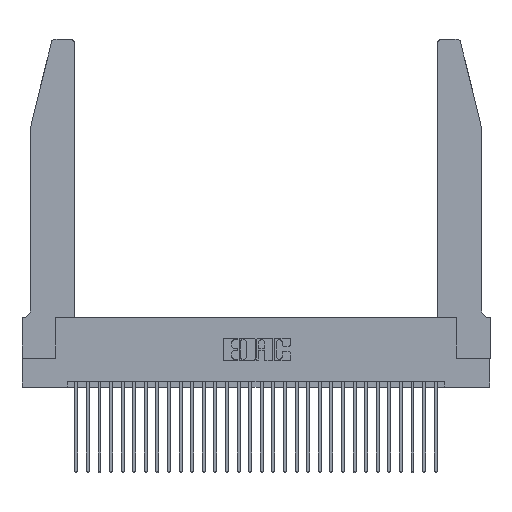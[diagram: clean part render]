
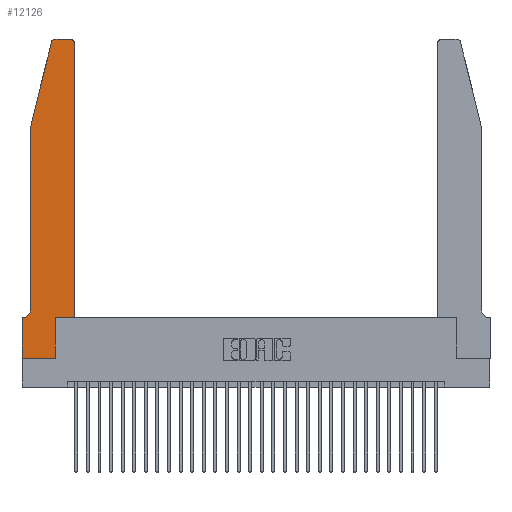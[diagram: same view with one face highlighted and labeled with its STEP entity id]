
A CAD part, top view. The second image highlights one B-rep face of the part: STEP entity #12126.
In plain terms, the highlighted planar face has unit normal (0, 0, 1).
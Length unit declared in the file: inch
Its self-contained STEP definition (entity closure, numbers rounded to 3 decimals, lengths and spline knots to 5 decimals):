
#45 = DIRECTION ( 'NONE',  ( 1., 0., 0. ) ) ;
#242 = DIRECTION ( 'NONE',  ( 1., 0., 0. ) ) ;
#439 = CARTESIAN_POINT ( 'NONE',  ( 0., 0., 0.37 ) ) ;
#577 = CARTESIAN_POINT ( 'NONE',  ( 0.0755, 0.35, 0.37 ) ) ;
#1180 = LINE ( 'NONE', #14344, #19770 ) ;
#1214 = EDGE_CURVE ( 'NONE', #13601, #24183, #5339, .T. ) ;
#1487 = CARTESIAN_POINT ( 'NONE',  ( 0.0755, 2., 0.37 ) ) ;
#1635 = CARTESIAN_POINT ( 'NONE',  ( 0.4205, 2.72, 0.37 ) ) ;
#1815 = EDGE_CURVE ( 'NONE', #28542, #14174, #22331, .T. ) ;
#2002 = EDGE_CURVE ( 'NONE', #27804, #28542, #4915, .T. ) ;
#2215 = CARTESIAN_POINT ( 'NONE',  ( 0.25487, 2.72718, 0.37 ) ) ;
#2487 = ORIENTED_EDGE ( 'NONE', *, *, #30683, .T. ) ;
#2909 = DIRECTION ( 'NONE',  ( 0., -1., 0. ) ) ;
#3044 = LINE ( 'NONE', #439, #27977 ) ;
#3140 = CARTESIAN_POINT ( 'NONE',  ( 0.2605, 2.75, 0.37 ) ) ;
#3738 = ORIENTED_EDGE ( 'NONE', *, *, #28276, .T. ) ;
#3820 = FACE_OUTER_BOUND ( 'NONE', #18249, .T. ) ;
#4070 = ORIENTED_EDGE ( 'NONE', *, *, #11507, .T. ) ;
#4106 = DIRECTION ( 'NONE',  ( 1., 0., 0. ) ) ;
#4196 = LINE ( 'NONE', #3140, #22747 ) ;
#4547 = CARTESIAN_POINT ( 'NONE',  ( 0.4505, 0.35, 0.37 ) ) ;
#4696 = VERTEX_POINT ( 'NONE', #9261 ) ;
#4725 = DIRECTION ( 'NONE',  ( 1., 0., 0. ) ) ;
#4732 = AXIS2_PLACEMENT_3D ( 'NONE', #1635, #18627, #4106 ) ;
#4915 = LINE ( 'NONE', #17251, #10599 ) ;
#5339 = LINE ( 'NONE', #577, #30224 ) ;
#5496 = CARTESIAN_POINT ( 'NONE',  ( 0.2865, 0.35, 0.37 ) ) ;
#5604 = DIRECTION ( 'NONE',  ( -1., 0., 0. ) ) ;
#5750 = CARTESIAN_POINT ( 'NONE',  ( 0.0055, 0.42, 0.37 ) ) ;
#5831 = EDGE_CURVE ( 'NONE', #15368, #27804, #14649, .T. ) ;
#6042 = LINE ( 'NONE', #22876, #18156 ) ;
#6234 = CARTESIAN_POINT ( 'NONE',  ( 0.4505, 2.72, 0.37 ) ) ;
#6347 = AXIS2_PLACEMENT_3D ( 'NONE', #5750, #22673, #8168 ) ;
#6459 = CIRCLE ( 'NONE', #11111, 0.03 ) ;
#6578 = CARTESIAN_POINT ( 'NONE',  ( 0.284, 2.75, 0.37 ) ) ;
#6589 = ORIENTED_EDGE ( 'NONE', *, *, #22868, .T. ) ;
#7071 = DIRECTION ( 'NONE',  ( 1., 0., 0. ) ) ;
#8168 = DIRECTION ( 'NONE',  ( -1., 0., 0. ) ) ;
#8858 = VERTEX_POINT ( 'NONE', #23568 ) ;
#9261 = CARTESIAN_POINT ( 'NONE',  ( 0., 0., 0.37 ) ) ;
#9435 = CARTESIAN_POINT ( 'NONE',  ( 0.0755, 2., 0.37 ) ) ;
#10599 = VECTOR ( 'NONE', #242, 39.37008 ) ;
#10813 = ORIENTED_EDGE ( 'NONE', *, *, #26811, .T. ) ;
#11095 = ORIENTED_EDGE ( 'NONE', *, *, #20569, .T. ) ;
#11111 = AXIS2_PLACEMENT_3D ( 'NONE', #29006, #14664, #45 ) ;
#11507 = EDGE_CURVE ( 'NONE', #4696, #15368, #1180, .T. ) ;
#11554 = CARTESIAN_POINT ( 'NONE',  ( 0.2865, 0.35, 0.37 ) ) ;
#11867 = DIRECTION ( 'NONE',  ( 0., 1., 0. ) ) ;
#11903 = VERTEX_POINT ( 'NONE', #17970 ) ;
#11948 = ORIENTED_EDGE ( 'NONE', *, *, #5831, .T. ) ;
#12126 = ADVANCED_FACE ( 'NONE', ( #3820 ), #31122, .T. ) ;
#12218 = CIRCLE ( 'NONE', #4732, 0.03 ) ;
#13289 = EDGE_CURVE ( 'NONE', #11903, #13601, #16708, .T. ) ;
#13530 = VERTEX_POINT ( 'NONE', #6578 ) ;
#13601 = VERTEX_POINT ( 'NONE', #30769 ) ;
#13670 = VERTEX_POINT ( 'NONE', #9435 ) ;
#13683 = VERTEX_POINT ( 'NONE', #2215 ) ;
#14019 = DIRECTION ( 'NONE',  ( 0., 1., 0. ) ) ;
#14174 = VERTEX_POINT ( 'NONE', #6234 ) ;
#14344 = CARTESIAN_POINT ( 'NONE',  ( 0., 0., 0.37 ) ) ;
#14649 = LINE ( 'NONE', #11554, #26639 ) ;
#14664 = DIRECTION ( 'NONE',  ( 0., 0., 1. ) ) ;
#14935 = ORIENTED_EDGE ( 'NONE', *, *, #2002, .T. ) ;
#15368 = VERTEX_POINT ( 'NONE', #26002 ) ;
#15793 = CARTESIAN_POINT ( 'NONE',  ( 0., 0.35, 0.37 ) ) ;
#16708 = CIRCLE ( 'NONE', #6347, 0.07 ) ;
#16811 = CARTESIAN_POINT ( 'NONE',  ( 0., 0.35, 0.37 ) ) ;
#17030 = ORIENTED_EDGE ( 'NONE', *, *, #1815, .T. ) ;
#17251 = CARTESIAN_POINT ( 'NONE',  ( 0.4505, 0.35, 0.37 ) ) ;
#17409 = ORIENTED_EDGE ( 'NONE', *, *, #29097, .T. ) ;
#17970 = CARTESIAN_POINT ( 'NONE',  ( 0.0755, 0.42, 0.37 ) ) ;
#18156 = VECTOR ( 'NONE', #25290, 39.37008 ) ;
#18249 = EDGE_LOOP ( 'NONE', ( #11095, #2487, #17409, #6589, #27532, #27013, #3738, #4070, #11948, #14935, #17030, #10813 ) ) ;
#18627 = DIRECTION ( 'NONE',  ( 0., 0., 1. ) ) ;
#19226 = DIRECTION ( 'NONE',  ( 0., 0., 1. ) ) ;
#19770 = VECTOR ( 'NONE', #7071, 39.37008 ) ;
#20112 = AXIS2_PLACEMENT_3D ( 'NONE', #16811, #19226, #4725 ) ;
#20569 = EDGE_CURVE ( 'NONE', #8858, #13530, #4196, .T. ) ;
#20889 = DIRECTION ( 'NONE',  ( 0., -1., 0. ) ) ;
#21569 = VECTOR ( 'NONE', #11867, 39.37008 ) ;
#22111 = DIRECTION ( 'NONE',  ( -1., 0., 0. ) ) ;
#22331 = LINE ( 'NONE', #4547, #21569 ) ;
#22673 = DIRECTION ( 'NONE',  ( 0., 0., -1. ) ) ;
#22747 = VECTOR ( 'NONE', #5604, 39.37008 ) ;
#22868 = EDGE_CURVE ( 'NONE', #13670, #11903, #30844, .T. ) ;
#22876 = CARTESIAN_POINT ( 'NONE',  ( 0.0755, 2., 0.37 ) ) ;
#23568 = CARTESIAN_POINT ( 'NONE',  ( 0.4205, 2.75, 0.37 ) ) ;
#24183 = VERTEX_POINT ( 'NONE', #15793 ) ;
#25290 = DIRECTION ( 'NONE',  ( -0.239, -0.971, 0. ) ) ;
#26002 = CARTESIAN_POINT ( 'NONE',  ( 0.2865, 0., 0.37 ) ) ;
#26639 = VECTOR ( 'NONE', #14019, 39.37008 ) ;
#26811 = EDGE_CURVE ( 'NONE', #14174, #8858, #12218, .T. ) ;
#27013 = ORIENTED_EDGE ( 'NONE', *, *, #1214, .T. ) ;
#27532 = ORIENTED_EDGE ( 'NONE', *, *, #13289, .T. ) ;
#27804 = VERTEX_POINT ( 'NONE', #5496 ) ;
#27977 = VECTOR ( 'NONE', #2909, 39.37008 ) ;
#28276 = EDGE_CURVE ( 'NONE', #24183, #4696, #3044, .T. ) ;
#28542 = VERTEX_POINT ( 'NONE', #30316 ) ;
#29006 = CARTESIAN_POINT ( 'NONE',  ( 0.284, 2.72, 0.37 ) ) ;
#29097 = EDGE_CURVE ( 'NONE', #13683, #13670, #6042, .T. ) ;
#30135 = VECTOR ( 'NONE', #20889, 39.37008 ) ;
#30224 = VECTOR ( 'NONE', #22111, 39.37008 ) ;
#30316 = CARTESIAN_POINT ( 'NONE',  ( 0.4505, 0.35, 0.37 ) ) ;
#30683 = EDGE_CURVE ( 'NONE', #13530, #13683, #6459, .T. ) ;
#30769 = CARTESIAN_POINT ( 'NONE',  ( 0.0055, 0.35, 0.37 ) ) ;
#30844 = LINE ( 'NONE', #1487, #30135 ) ;
#31122 = PLANE ( 'NONE',  #20112 ) ;
